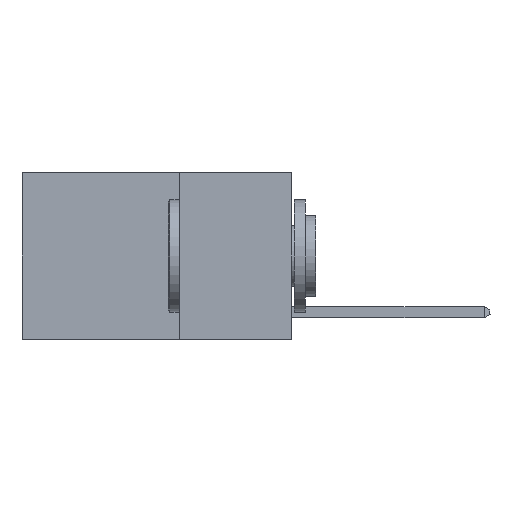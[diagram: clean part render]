
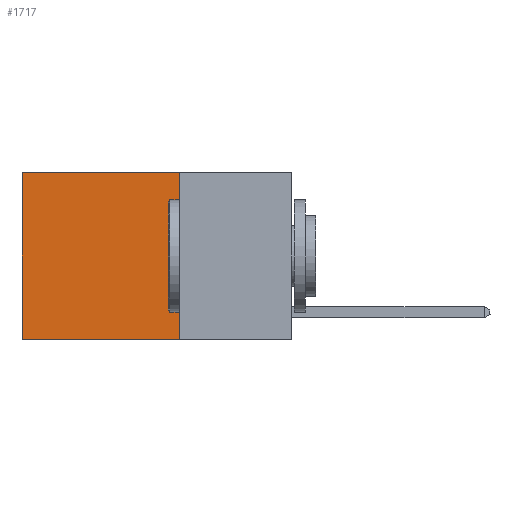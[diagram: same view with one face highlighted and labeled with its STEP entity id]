
A CAD part, left-side view. The second image highlights one B-rep face of the part: STEP entity #1717.
In plain terms, the highlighted planar face has unit normal (-1, 0, 0).
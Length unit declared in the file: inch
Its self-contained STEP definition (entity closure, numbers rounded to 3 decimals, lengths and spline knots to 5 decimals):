
#146 = ORIENTED_EDGE ( 'NONE', *, *, #8757, .F. ) ;
#242 = CARTESIAN_POINT ( 'NONE',  ( 0.2625, 0.6, 0. ) ) ;
#311 = EDGE_CURVE ( 'NONE', #6965, #8951, #12334, .T. ) ;
#524 = DIRECTION ( 'NONE',  ( 0., 1., 0. ) ) ;
#1717 = ADVANCED_FACE ( 'NONE', ( #12612 ), #12691, .F. ) ;
#1758 = CARTESIAN_POINT ( 'NONE',  ( 0.2625, 0.25, 0. ) ) ;
#1850 = VECTOR ( 'NONE', #9985, 39.37008 ) ;
#1853 = DIRECTION ( 'NONE',  ( 1., 0., 0. ) ) ;
#3754 = CARTESIAN_POINT ( 'NONE',  ( 0.2625, 0.25, 0. ) ) ;
#4036 = ORIENTED_EDGE ( 'NONE', *, *, #311, .T. ) ;
#4493 = ORIENTED_EDGE ( 'NONE', *, *, #8580, .T. ) ;
#5102 = LINE ( 'NONE', #12389, #11034 ) ;
#5487 = VECTOR ( 'NONE', #9544, 39.37008 ) ;
#5634 = CARTESIAN_POINT ( 'NONE',  ( 0.2625, 0.25, 0. ) ) ;
#6146 = DIRECTION ( 'NONE',  ( 0., 1., 0. ) ) ;
#6965 = VERTEX_POINT ( 'NONE', #242 ) ;
#7083 = LINE ( 'NONE', #3754, #12520 ) ;
#8069 = DIRECTION ( 'NONE',  ( 0., 0., -1. ) ) ;
#8353 = CARTESIAN_POINT ( 'NONE',  ( 0.2625, 0.25, 0. ) ) ;
#8580 = EDGE_CURVE ( 'NONE', #11716, #6965, #7083, .T. ) ;
#8757 = EDGE_CURVE ( 'NONE', #8799, #8951, #5102, .T. ) ;
#8799 = VERTEX_POINT ( 'NONE', #10125 ) ;
#8951 = VERTEX_POINT ( 'NONE', #9101 ) ;
#9101 = CARTESIAN_POINT ( 'NONE',  ( 0.2625, 0.6, -0.37 ) ) ;
#9108 = ORIENTED_EDGE ( 'NONE', *, *, #9396, .F. ) ;
#9159 = AXIS2_PLACEMENT_3D ( 'NONE', #5634, #1853, #8069 ) ;
#9396 = EDGE_CURVE ( 'NONE', #11716, #8799, #10485, .T. ) ;
#9544 = DIRECTION ( 'NONE',  ( 0., 0., -1. ) ) ;
#9985 = DIRECTION ( 'NONE',  ( 0., 0., -1. ) ) ;
#10125 = CARTESIAN_POINT ( 'NONE',  ( 0.2625, 0.25, -0.37 ) ) ;
#10485 = LINE ( 'NONE', #8353, #5487 ) ;
#11034 = VECTOR ( 'NONE', #524, 39.37008 ) ;
#11716 = VERTEX_POINT ( 'NONE', #1758 ) ;
#12183 = CARTESIAN_POINT ( 'NONE',  ( 0.2625, 0.6, 0. ) ) ;
#12334 = LINE ( 'NONE', #12183, #1850 ) ;
#12389 = CARTESIAN_POINT ( 'NONE',  ( 0.2625, 0.25, -0.37 ) ) ;
#12520 = VECTOR ( 'NONE', #6146, 39.37008 ) ;
#12612 = FACE_OUTER_BOUND ( 'NONE', #14736, .T. ) ;
#12691 = PLANE ( 'NONE',  #9159 ) ;
#14736 = EDGE_LOOP ( 'NONE', ( #4036, #146, #9108, #4493 ) ) ;
